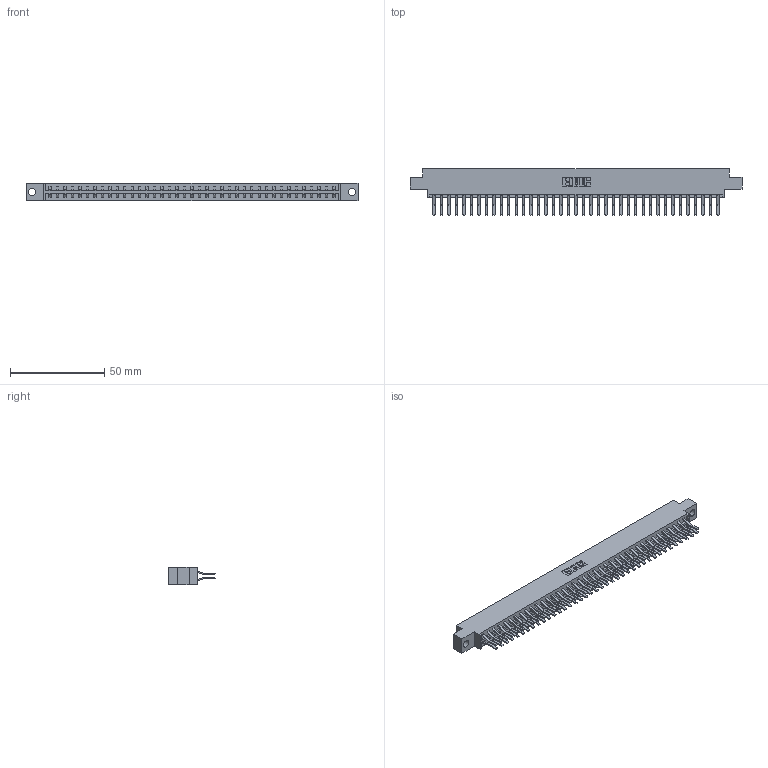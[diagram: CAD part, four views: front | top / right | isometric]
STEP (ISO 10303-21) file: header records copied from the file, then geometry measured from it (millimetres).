
FILE_DESCRIPTION (( 'STEP AP203' ), '1' );
FILE_NAME ('833-078-560-804.STEP', '2020-06-05T21:02:21', ( '' ), ( '' ), 'SwSTEP 2.0', 'SolidWorks 2020', '' );
FILE_SCHEMA (( 'CONFIG_CONTROL_DESIGN' ));
Length unit declared in the file: inch
Products named in the file (3): 833-078-560-804; 345-292-001_560 Tail; 833 Part_Offset - .156 Dia - TH
Assembly tree (79 placements, depth 2):
  833-078-560-804
    833 Part_Offset - .156 Dia - TH
    345-292-001_560 Tail  x78
Bounding box: 176.07 x 24.78 x 9.4 mm (x, y, z)
Volume: 18143.6 mm3; surface area: 22896.7 mm2
Topology: 79 solids, 79 shells, 4330 faces, 12881 edges, 8482 vertices
Faces by surface type: plane 2882, cylinder 1448
Entity records: 25701 total; most frequent: CARTESIAN_POINT 4266, ORIENTED_EDGE 4202, DIRECTION 3653, EDGE_CURVE 2101, LINE 1969, VECTOR 1969, VERTEX_POINT 1398, AXIS2_PLACEMENT_3D 842
